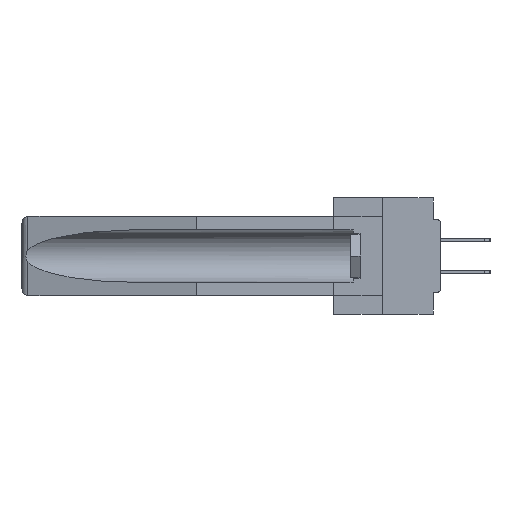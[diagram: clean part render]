
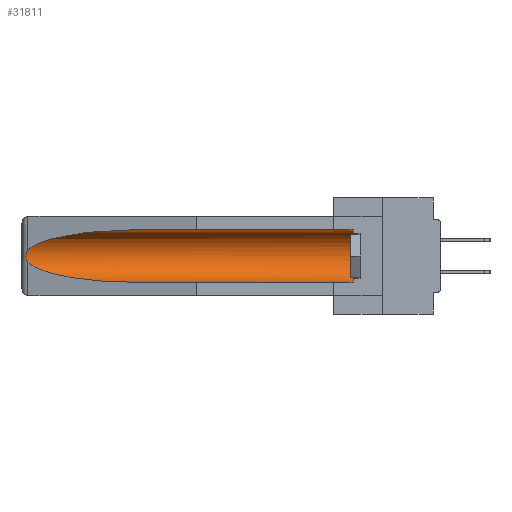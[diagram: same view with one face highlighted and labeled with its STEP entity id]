
A CAD part, left-side view. The second image highlights one B-rep face of the part: STEP entity #31811.
In plain terms, the highlighted cylindrical face has radius 2.857 mm (diameter 5.715 mm), a partial arc.
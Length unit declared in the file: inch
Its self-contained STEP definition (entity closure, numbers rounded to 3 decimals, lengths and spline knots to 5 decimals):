
#1956 = DIRECTION ( 'NONE',  ( 0., 0., 1. ) ) ;
#2184 = ORIENTED_EDGE ( 'NONE', *, *, #3080, .T. ) ;
#2531 = CARTESIAN_POINT ( 'NONE',  ( 0.26597, 1.5296, -0.19026 ) ) ;
#3080 = EDGE_CURVE ( 'NONE', #20430, #13657, #16600, .T. ) ;
#3557 = VERTEX_POINT ( 'NONE', #15409 ) ;
#3749 = CARTESIAN_POINT ( 'NONE',  ( 0.26537, 1.52718, -0.14972 ) ) ;
#4223 = CIRCLE ( 'NONE', #39135, 0.1125 ) ;
#4236 = VERTEX_POINT ( 'NONE', #20746 ) ;
#4731 = DIRECTION ( 'NONE',  ( 0., 1., 0. ) ) ;
#4965 =( BOUNDED_CURVE ( )  B_SPLINE_CURVE ( 3, ( #16014, #34158, #30945, #3749 ),
 .UNSPECIFIED., .F., .T. ) 
 B_SPLINE_CURVE_WITH_KNOTS ( ( 4, 4 ),
 ( 4.71239, 6.08839 ),
 .UNSPECIFIED. ) 
 CURVE ( )  GEOMETRIC_REPRESENTATION_ITEM ( )  RATIONAL_B_SPLINE_CURVE ( ( 1., 0.848, 0.848, 1. ) ) 
 REPRESENTATION_ITEM ( '' )  );
#5246 = CARTESIAN_POINT ( 'NONE',  ( 0.26537, 1.52718, -0.14972 ) ) ;
#6939 = ORIENTED_EDGE ( 'NONE', *, *, #37850, .F. ) ;
#7081 = CARTESIAN_POINT ( 'NONE',  ( 0.26537, 1.52718, -0.19328 ) ) ;
#7483 = CYLINDRICAL_SURFACE ( 'NONE', #28782, 0.1125 ) ;
#9704 = VERTEX_POINT ( 'NONE', #29474 ) ;
#9828 = CARTESIAN_POINT ( 'NONE',  ( 0.155, -0.30754, -0.059 ) ) ;
#10521 = EDGE_CURVE ( 'NONE', #13657, #24097, #19020, .T. ) ;
#10882 = DIRECTION ( 'NONE',  ( 0., 0., 1. ) ) ;
#10895 = CARTESIAN_POINT ( 'NONE',  ( 0.21114, 1.30732, -0.284 ) ) ;
#11533 = CARTESIAN_POINT ( 'NONE',  ( 0.2673, 1.5327, -0.16383 ) ) ;
#11670 = CARTESIAN_POINT ( 'NONE',  ( 0.26597, 1.52961, -0.15275 ) ) ;
#12474 = EDGE_CURVE ( 'NONE', #9704, #4236, #31984, .T. ) ;
#13587 = ORIENTED_EDGE ( 'NONE', *, *, #12474, .T. ) ;
#13657 = VERTEX_POINT ( 'NONE', #17356 ) ;
#14053 = LINE ( 'NONE', #36011, #32968 ) ;
#15409 = CARTESIAN_POINT ( 'NONE',  ( 0.155, 0.126, -0.284 ) ) ;
#16014 = CARTESIAN_POINT ( 'NONE',  ( 0.155, 1.07973, -0.059 ) ) ;
#16600 = B_SPLINE_CURVE_WITH_KNOTS ( 'NONE', 3,
 ( #23256, #11670, #23766, #11533, #35567, #29331, #26581, #38362, #2531, #17461 ),
 .UNSPECIFIED., .F., .F.,
 ( 4, 2, 2, 2, 4 ),
 ( 0., 0.00029, 0.00058, 0.00087, 0.00117 ),
 .UNSPECIFIED. ) ;
#17356 = CARTESIAN_POINT ( 'NONE',  ( 0.26537, 1.52718, -0.19328 ) ) ;
#17461 = CARTESIAN_POINT ( 'NONE',  ( 0.26537, 1.52718, -0.19328 ) ) ;
#17623 = DIRECTION ( 'NONE',  ( 0., 1., 0. ) ) ;
#19020 =( BOUNDED_CURVE ( )  B_SPLINE_CURVE ( 3, ( #7081, #37318, #10895, #23260 ),
 .UNSPECIFIED., .F., .F. ) 
 B_SPLINE_CURVE_WITH_KNOTS ( ( 4, 4 ),
 ( 0.1948, 1.5708 ),
 .UNSPECIFIED. ) 
 CURVE ( )  GEOMETRIC_REPRESENTATION_ITEM ( )  RATIONAL_B_SPLINE_CURVE ( ( 1., 0.848, 0.848, 1. ) ) 
 REPRESENTATION_ITEM ( '' )  );
#20430 = VERTEX_POINT ( 'NONE', #5246 ) ;
#20746 = CARTESIAN_POINT ( 'NONE',  ( 0.155, 1.07973, -0.059 ) ) ;
#21266 = EDGE_LOOP ( 'NONE', ( #34839, #2184, #33344, #6939, #36697, #13587 ) ) ;
#21517 = DIRECTION ( 'NONE',  ( 0., 1., 0. ) ) ;
#23256 = CARTESIAN_POINT ( 'NONE',  ( 0.26537, 1.52718, -0.14972 ) ) ;
#23260 = CARTESIAN_POINT ( 'NONE',  ( 0.155, 1.07973, -0.284 ) ) ;
#23766 = CARTESIAN_POINT ( 'NONE',  ( 0.26654, 1.53092, -0.15636 ) ) ;
#24097 = VERTEX_POINT ( 'NONE', #29667 ) ;
#26581 = CARTESIAN_POINT ( 'NONE',  ( 0.2673, 1.53269, -0.17917 ) ) ;
#28201 = EDGE_CURVE ( 'NONE', #4236, #20430, #4965, .T. ) ;
#28297 = EDGE_CURVE ( 'NONE', #3557, #9704, #4223, .T. ) ;
#28420 = DIRECTION ( 'NONE',  ( 0., -1., 0. ) ) ;
#28782 = AXIS2_PLACEMENT_3D ( 'NONE', #35114, #4731, #1956 ) ;
#29331 = CARTESIAN_POINT ( 'NONE',  ( 0.2675, 1.53308, -0.17534 ) ) ;
#29474 = CARTESIAN_POINT ( 'NONE',  ( 0.155, 0.126, -0.059 ) ) ;
#29667 = CARTESIAN_POINT ( 'NONE',  ( 0.155, 1.07973, -0.284 ) ) ;
#30945 = CARTESIAN_POINT ( 'NONE',  ( 0.25451, 1.48313, -0.09465 ) ) ;
#30970 = VECTOR ( 'NONE', #21517, 39.37008 ) ;
#31811 = ADVANCED_FACE ( 'NONE', ( #38653 ), #7483, .F. ) ;
#31984 = LINE ( 'NONE', #9828, #30970 ) ;
#32968 = VECTOR ( 'NONE', #17623, 39.37008 ) ;
#33344 = ORIENTED_EDGE ( 'NONE', *, *, #10521, .T. ) ;
#34158 = CARTESIAN_POINT ( 'NONE',  ( 0.21114, 1.30732, -0.059 ) ) ;
#34839 = ORIENTED_EDGE ( 'NONE', *, *, #28201, .T. ) ;
#35114 = CARTESIAN_POINT ( 'NONE',  ( 0.155, -0.30754, -0.1715 ) ) ;
#35567 = CARTESIAN_POINT ( 'NONE',  ( 0.2675, 1.53308, -0.16763 ) ) ;
#36011 = CARTESIAN_POINT ( 'NONE',  ( 0.155, -0.30754, -0.284 ) ) ;
#36697 = ORIENTED_EDGE ( 'NONE', *, *, #28297, .T. ) ;
#37318 = CARTESIAN_POINT ( 'NONE',  ( 0.25451, 1.48313, -0.24835 ) ) ;
#37834 = CARTESIAN_POINT ( 'NONE',  ( 0.155, 0.126, -0.1715 ) ) ;
#37850 = EDGE_CURVE ( 'NONE', #3557, #24097, #14053, .T. ) ;
#38362 = CARTESIAN_POINT ( 'NONE',  ( 0.26655, 1.53094, -0.18657 ) ) ;
#38653 = FACE_OUTER_BOUND ( 'NONE', #21266, .T. ) ;
#39135 = AXIS2_PLACEMENT_3D ( 'NONE', #37834, #28420, #10882 ) ;
